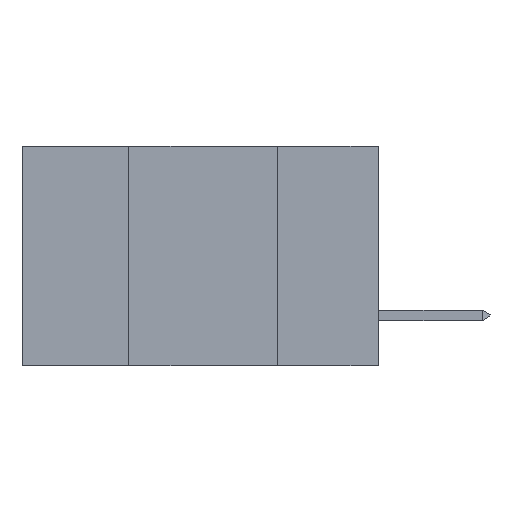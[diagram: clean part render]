
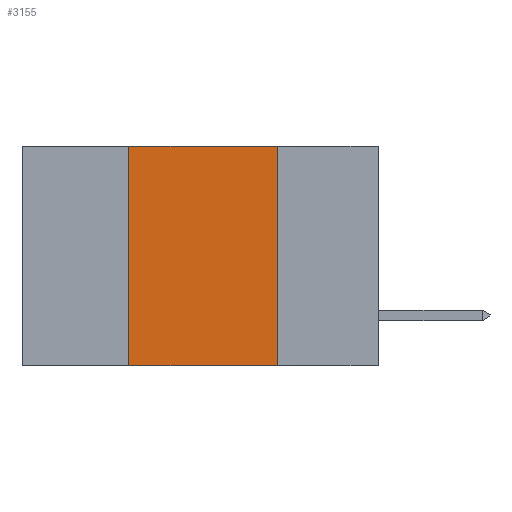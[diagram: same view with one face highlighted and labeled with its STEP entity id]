
A CAD part, left-side view. The second image highlights one B-rep face of the part: STEP entity #3155.
In plain terms, the highlighted planar face has unit normal (-1, 0, 0).
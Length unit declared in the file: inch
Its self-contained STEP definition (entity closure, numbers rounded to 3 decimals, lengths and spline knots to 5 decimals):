
#634 = VERTEX_POINT ( 'NONE', #16900 ) ;
#2715 = LINE ( 'NONE', #17788, #16997 ) ;
#3155 = ADVANCED_FACE ( 'NONE', ( #4415 ), #17632, .F. ) ;
#4151 = VERTEX_POINT ( 'NONE', #4875 ) ;
#4415 = FACE_OUTER_BOUND ( 'NONE', #17314, .T. ) ;
#4429 = EDGE_CURVE ( 'NONE', #4151, #20542, #11180, .T. ) ;
#4630 = DIRECTION ( 'NONE',  ( 0., 0., 1. ) ) ;
#4875 = CARTESIAN_POINT ( 'NONE',  ( 0., 0.42, -0.37 ) ) ;
#5870 = VERTEX_POINT ( 'NONE', #12334 ) ;
#5897 = EDGE_CURVE ( 'NONE', #20542, #634, #7552, .T. ) ;
#5906 = CARTESIAN_POINT ( 'NONE',  ( 0., 0.6, 0. ) ) ;
#7552 = LINE ( 'NONE', #5906, #14347 ) ;
#7590 = DIRECTION ( 'NONE',  ( 1., 0., 0. ) ) ;
#7702 = CARTESIAN_POINT ( 'NONE',  ( 0., 0.42, -0.37 ) ) ;
#8699 = DIRECTION ( 'NONE',  ( 0., -1., 0. ) ) ;
#9395 = DIRECTION ( 'NONE',  ( 0., 0., -1. ) ) ;
#9731 = ORIENTED_EDGE ( 'NONE', *, *, #18242, .F. ) ;
#11085 = ORIENTED_EDGE ( 'NONE', *, *, #14751, .T. ) ;
#11180 = LINE ( 'NONE', #7702, #14690 ) ;
#12056 = VECTOR ( 'NONE', #8699, 39.37008 ) ;
#12259 = AXIS2_PLACEMENT_3D ( 'NONE', #16318, #7590, #12696 ) ;
#12334 = CARTESIAN_POINT ( 'NONE',  ( 0., 0.17, -0.37 ) ) ;
#12696 = DIRECTION ( 'NONE',  ( 0., 0., -1. ) ) ;
#14197 = DIRECTION ( 'NONE',  ( 0., -1., 0. ) ) ;
#14347 = VECTOR ( 'NONE', #14197, 39.37008 ) ;
#14690 = VECTOR ( 'NONE', #4630, 39.37008 ) ;
#14751 = EDGE_CURVE ( 'NONE', #4151, #5870, #18641, .T. ) ;
#15473 = ORIENTED_EDGE ( 'NONE', *, *, #5897, .F. ) ;
#16318 = CARTESIAN_POINT ( 'NONE',  ( 0., 0.6, 0. ) ) ;
#16900 = CARTESIAN_POINT ( 'NONE',  ( 0., 0.17, 0. ) ) ;
#16986 = CARTESIAN_POINT ( 'NONE',  ( 0., 0.6, -0.37 ) ) ;
#16997 = VECTOR ( 'NONE', #9395, 39.37008 ) ;
#17314 = EDGE_LOOP ( 'NONE', ( #9731, #15473, #19626, #11085 ) ) ;
#17632 = PLANE ( 'NONE',  #12259 ) ;
#17788 = CARTESIAN_POINT ( 'NONE',  ( 0., 0.17, -0.37 ) ) ;
#18242 = EDGE_CURVE ( 'NONE', #634, #5870, #2715, .T. ) ;
#18641 = LINE ( 'NONE', #16986, #12056 ) ;
#19626 = ORIENTED_EDGE ( 'NONE', *, *, #4429, .F. ) ;
#20359 = CARTESIAN_POINT ( 'NONE',  ( 0., 0.42, 0. ) ) ;
#20542 = VERTEX_POINT ( 'NONE', #20359 ) ;
